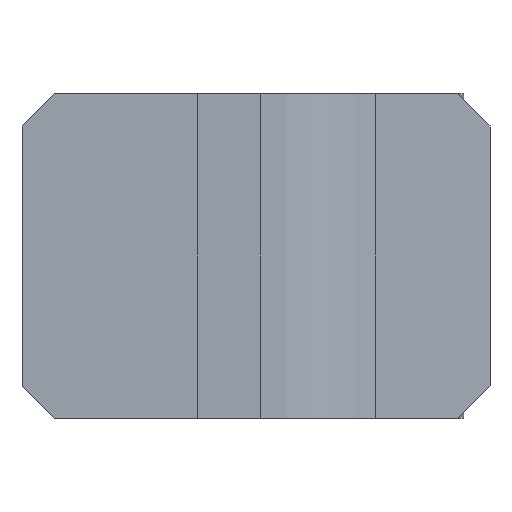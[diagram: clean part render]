
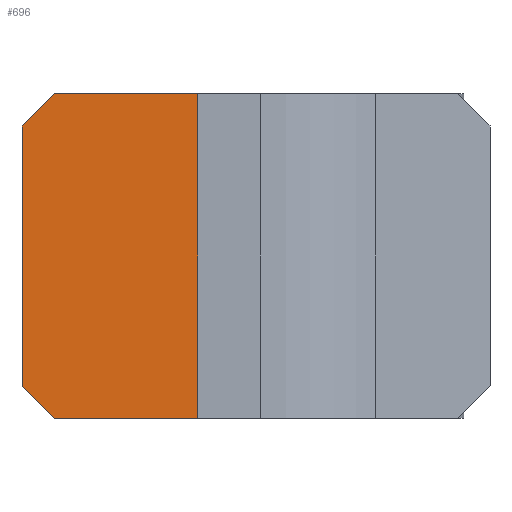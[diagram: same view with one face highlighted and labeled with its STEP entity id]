
A CAD part, left-side view. The second image highlights one B-rep face of the part: STEP entity #696.
In plain terms, the highlighted planar face has unit normal (-1, 0, 0).
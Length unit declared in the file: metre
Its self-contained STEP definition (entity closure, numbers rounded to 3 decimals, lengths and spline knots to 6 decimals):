
#119=ORIENTED_EDGE('',*,*,#311,.T.);
#120=ORIENTED_EDGE('',*,*,#312,.T.);
#121=ORIENTED_EDGE('',*,*,#310,.T.);
#122=ORIENTED_EDGE('',*,*,#313,.T.);
#123=ORIENTED_EDGE('',*,*,#314,.F.);
#124=ORIENTED_EDGE('',*,*,#315,.F.);
#310=EDGE_CURVE('',#395,#400,#470,.T.);
#311=EDGE_CURVE('',#401,#402,#471,.T.);
#312=EDGE_CURVE('',#402,#395,#472,.T.);
#313=EDGE_CURVE('',#400,#403,#473,.F.);
#314=EDGE_CURVE('',#404,#403,#474,.T.);
#315=EDGE_CURVE('',#401,#404,#475,.T.);
#395=VERTEX_POINT('',#1095);
#400=VERTEX_POINT('',#1104);
#401=VERTEX_POINT('',#1108);
#402=VERTEX_POINT('',#1109);
#403=VERTEX_POINT('',#1112);
#404=VERTEX_POINT('',#1114);
#470=LINE('',#1105,#544);
#471=LINE('',#1107,#545);
#472=LINE('',#1110,#546);
#473=LINE('',#1111,#547);
#474=LINE('',#1113,#548);
#475=LINE('',#1115,#549);
#544=VECTOR('',#891,1.);
#545=VECTOR('',#894,1.);
#546=VECTOR('',#895,1.);
#547=VECTOR('',#896,1.);
#548=VECTOR('',#897,1.);
#549=VECTOR('',#898,1.);
#596=EDGE_LOOP('',(#119,#120,#121,#122,#123,#124));
#636=FACE_BOUND('',#596,.T.);
#668=PLANE('',#758);
#696=ADVANCED_FACE('',(#636),#668,.T.);
#758=AXIS2_PLACEMENT_3D('',#1106,#892,#893);
#891=DIRECTION('',(0.,0.,-1.));
#892=DIRECTION('',(-1.,0.,0.));
#893=DIRECTION('',(0.,0.,1.));
#894=DIRECTION('',(0.,1.,0.));
#895=DIRECTION('',(0.,0.707,-0.707));
#896=DIRECTION('',(0.,0.707,0.707));
#897=DIRECTION('',(0.,1.,0.));
#898=DIRECTION('',(0.,0.,-1.));
#1095=CARTESIAN_POINT('',(-0.019343,0.001837,0.06285));
#1104=CARTESIAN_POINT('',(-0.019343,0.001837,0.05777));
#1105=CARTESIAN_POINT('',(-0.019343,0.001837,0.063485));
#1106=CARTESIAN_POINT('',(-0.019343,0.000123,0.063485));
#1107=CARTESIAN_POINT('',(-0.019343,0.000123,0.063485));
#1108=CARTESIAN_POINT('',(-0.019343,-0.001592,0.063485));
#1109=CARTESIAN_POINT('',(-0.019343,0.001202,0.063485));
#1110=CARTESIAN_POINT('',(-0.019343,0.000662,0.064024));
#1111=CARTESIAN_POINT('',(-0.019343,0.003837,0.05977));
#1112=CARTESIAN_POINT('',(-0.019343,0.001202,0.057135));
#1113=CARTESIAN_POINT('',(-0.019343,0.000123,0.057135));
#1114=CARTESIAN_POINT('',(-0.019343,-0.001592,0.057135));
#1115=CARTESIAN_POINT('',(-0.019343,-0.001592,0.063485));
